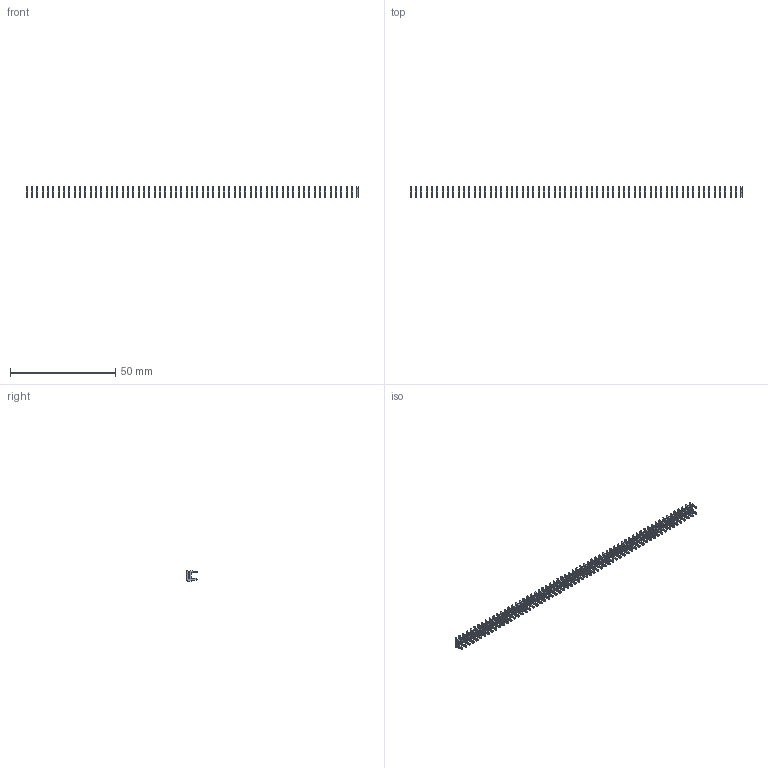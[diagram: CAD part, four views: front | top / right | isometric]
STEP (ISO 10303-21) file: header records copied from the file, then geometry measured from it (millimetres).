
FILE_DESCRIPTION (( 'STEP AP203' ), '1' );
FILE_NAME ('105-063-208-100.STEP', '2020-04-08T00:59:04', ( '' ), ( '' ), 'SwSTEP 2.0', 'SolidWorks 2016', '' );
FILE_SCHEMA (( 'CONFIG_CONTROL_DESIGN' ));
Length unit declared in the file: inch
Products named in the file (2): 105-063-208-100; 100-290-001_100-290-208
Assembly tree (63 placements, depth 2):
  105-063-208-100
    100-290-001_100-290-208  x63
Bounding box: 157.99 x 4.83 x 5.17 mm (x, y, z)
Volume: 433.5 mm3; surface area: 2677.3 mm2
Topology: 63 solids, 63 shells, 1575 faces, 4347 edges, 2898 vertices
Faces by surface type: plane 1386, cylinder 189
Entity records: 2973 total; most frequent: DIRECTION 257, CARTESIAN_POINT 206, ORIENTED_EDGE 138, LOCAL_TIME 136, CALENDAR_DATE 136, DATE_AND_TIME 136, COORDINATED_UNIVERSAL_TIME_OFFSET 136, AXIS2_PLACEMENT_3D 97
